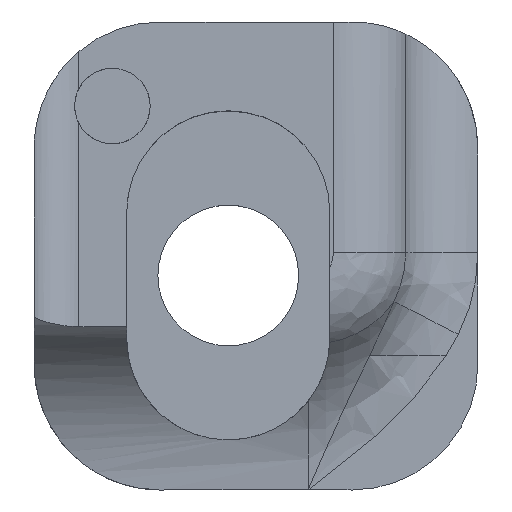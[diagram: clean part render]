
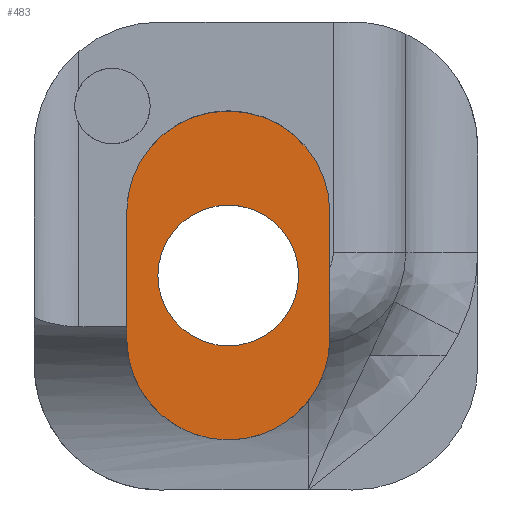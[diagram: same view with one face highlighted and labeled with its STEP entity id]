
A CAD part, top view. The second image highlights one B-rep face of the part: STEP entity #483.
In plain terms, the highlighted planar face has unit normal (0, 0, 1).
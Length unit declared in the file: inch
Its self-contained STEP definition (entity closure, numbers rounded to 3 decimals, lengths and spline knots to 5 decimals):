
#16 = CARTESIAN_POINT ( 'NONE',  ( 3.23644, 2.08681, 7.74339 ) ) ;
#23 = CARTESIAN_POINT ( 'NONE',  ( 3.23644, 2.45455, 7.74339 ) ) ;
#178 = DIRECTION ( 'NONE',  ( 0., -1., 0. ) ) ;
#181 = DIRECTION ( 'NONE',  ( 0., 0., 1. ) ) ;
#182 = CARTESIAN_POINT ( 'NONE',  ( 3.23644, 2.24581, 7.74339 ) ) ;
#198 = DIRECTION ( 'NONE',  ( 0., 1., 0. ) ) ;
#204 = CARTESIAN_POINT ( 'NONE',  ( 3.39544, 2.24581, 7.74339 ) ) ;
#280 = EDGE_CURVE ( 'NONE', #1385, #627, #694, .T. ) ;
#285 = EDGE_CURVE ( 'NONE', #1067, #1385, #995, .T. ) ;
#287 = DIRECTION ( 'NONE',  ( 0., -1., 0. ) ) ;
#289 = DIRECTION ( 'NONE',  ( 0., 0., 1. ) ) ;
#290 = EDGE_CURVE ( 'NONE', #784, #1067, #981, .T. ) ;
#295 = CARTESIAN_POINT ( 'NONE',  ( 3.23644, 2.44281, 7.74339 ) ) ;
#367 = DIRECTION ( 'NONE',  ( 0., -1., 0. ) ) ;
#380 = PLANE ( 'NONE',  #1120 ) ;
#393 = CARTESIAN_POINT ( 'NONE',  ( 3.23644, 2.44281, 7.74339 ) ) ;
#397 = CARTESIAN_POINT ( 'NONE',  ( 3.39544, 2.44281, 7.74339 ) ) ;
#454 = ORIENTED_EDGE ( 'NONE', *, *, #847, .F. ) ;
#455 = EDGE_CURVE ( 'NONE', #702, #469, #967, .T. ) ;
#458 = ORIENTED_EDGE ( 'NONE', *, *, #280, .T. ) ;
#469 = VERTEX_POINT ( 'NONE', #960 ) ;
#483 = ADVANCED_FACE ( 'NONE', ( #1066, #1369 ), #380, .T. ) ;
#491 = AXIS2_PLACEMENT_3D ( 'NONE', #182, #181, #178 ) ;
#495 = ORIENTED_EDGE ( 'NONE', *, *, #565, .T. ) ;
#521 = ORIENTED_EDGE ( 'NONE', *, *, #834, .T. ) ;
#522 = CARTESIAN_POINT ( 'NONE',  ( 3.07744, 2.24581, 7.74339 ) ) ;
#535 = ORIENTED_EDGE ( 'NONE', *, *, #290, .T. ) ;
#553 = ORIENTED_EDGE ( 'NONE', *, *, #285, .T. ) ;
#565 = EDGE_CURVE ( 'NONE', #627, #1240, #1287, .T. ) ;
#627 = VERTEX_POINT ( 'NONE', #1316 ) ;
#694 = CIRCLE ( 'NONE', #1010, 0.159 ) ;
#702 = VERTEX_POINT ( 'NONE', #23 ) ;
#709 = AXIS2_PLACEMENT_3D ( 'NONE', #977, #974, #971 ) ;
#717 = DIRECTION ( 'NONE',  ( 0., 0., 1. ) ) ;
#784 = VERTEX_POINT ( 'NONE', #16 ) ;
#834 = EDGE_CURVE ( 'NONE', #1240, #784, #876, .T. ) ;
#847 = EDGE_CURVE ( 'NONE', #469, #702, #879, .T. ) ;
#876 = CIRCLE ( 'NONE', #1263, 0.159 ) ;
#879 = CIRCLE ( 'NONE', #1102, 0.11024 ) ;
#892 = CARTESIAN_POINT ( 'NONE',  ( 3.39544, 2.24581, 7.74339 ) ) ;
#960 = CARTESIAN_POINT ( 'NONE',  ( 3.23644, 2.23407, 7.74339 ) ) ;
#967 = CIRCLE ( 'NONE', #709, 0.11024 ) ;
#971 = DIRECTION ( 'NONE',  ( 0., -1., 0. ) ) ;
#974 = DIRECTION ( 'NONE',  ( 0., 0., 1. ) ) ;
#977 = CARTESIAN_POINT ( 'NONE',  ( 3.23644, 2.34431, 7.74339 ) ) ;
#981 = CIRCLE ( 'NONE', #491, 0.159 ) ;
#995 = LINE ( 'NONE', #204, #1368 ) ;
#1010 = AXIS2_PLACEMENT_3D ( 'NONE', #295, #289, #287 ) ;
#1066 = FACE_BOUND ( 'NONE', #1194, .T. ) ;
#1067 = VERTEX_POINT ( 'NONE', #892 ) ;
#1089 = DIRECTION ( 'NONE',  ( 0., -1., 0. ) ) ;
#1096 = DIRECTION ( 'NONE',  ( 0., 0., 1. ) ) ;
#1101 = CARTESIAN_POINT ( 'NONE',  ( 3.23644, 2.34431, 7.74339 ) ) ;
#1102 = AXIS2_PLACEMENT_3D ( 'NONE', #1101, #1096, #1089 ) ;
#1120 = AXIS2_PLACEMENT_3D ( 'NONE', #393, #717, #367 ) ;
#1133 = ORIENTED_EDGE ( 'NONE', *, *, #455, .F. ) ;
#1148 = EDGE_LOOP ( 'NONE', ( #458, #495, #521, #535, #553 ) ) ;
#1194 = EDGE_LOOP ( 'NONE', ( #454, #1133 ) ) ;
#1198 = DIRECTION ( 'NONE',  ( 0., -1., 0. ) ) ;
#1210 = DIRECTION ( 'NONE',  ( 0., -1., 0. ) ) ;
#1213 = CARTESIAN_POINT ( 'NONE',  ( 3.07744, 2.44281, 7.74339 ) ) ;
#1218 = DIRECTION ( 'NONE',  ( 0., 0., 1. ) ) ;
#1224 = CARTESIAN_POINT ( 'NONE',  ( 3.23644, 2.24581, 7.74339 ) ) ;
#1239 = VECTOR ( 'NONE', #1198, 39.37008 ) ;
#1240 = VERTEX_POINT ( 'NONE', #522 ) ;
#1263 = AXIS2_PLACEMENT_3D ( 'NONE', #1224, #1218, #1210 ) ;
#1287 = LINE ( 'NONE', #1213, #1239 ) ;
#1316 = CARTESIAN_POINT ( 'NONE',  ( 3.07744, 2.44281, 7.74339 ) ) ;
#1368 = VECTOR ( 'NONE', #198, 39.37008 ) ;
#1369 = FACE_OUTER_BOUND ( 'NONE', #1148, .T. ) ;
#1385 = VERTEX_POINT ( 'NONE', #397 ) ;
